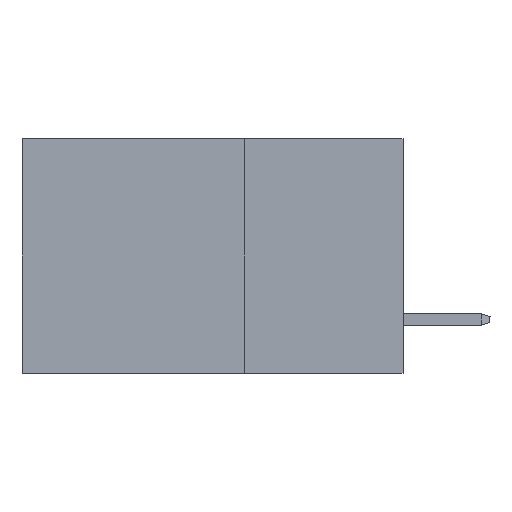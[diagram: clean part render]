
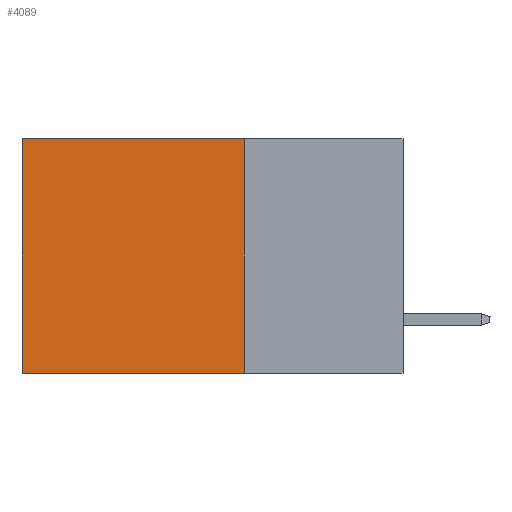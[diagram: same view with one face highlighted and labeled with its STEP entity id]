
A CAD part, left-side view. The second image highlights one B-rep face of the part: STEP entity #4089.
In plain terms, the highlighted planar face has unit normal (-1, 0, 0).
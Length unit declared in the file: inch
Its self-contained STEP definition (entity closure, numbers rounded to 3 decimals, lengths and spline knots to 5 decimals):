
#2768 = AXIS2_PLACEMENT_3D ( 'NONE', #8607, #30535, #14012 ) ;
#3609 = CARTESIAN_POINT ( 'NONE',  ( 0.2875, 0.6, 0. ) ) ;
#3750 = ORIENTED_EDGE ( 'NONE', *, *, #21855, .T. ) ;
#4089 = ADVANCED_FACE ( 'NONE', ( #13552 ), #20753, .F. ) ;
#5744 = CARTESIAN_POINT ( 'NONE',  ( 0.2875, 0.6, 0. ) ) ;
#6732 = CARTESIAN_POINT ( 'NONE',  ( 0.2875, 0.25, 0. ) ) ;
#8607 = CARTESIAN_POINT ( 'NONE',  ( 0.2875, 0.25, 0. ) ) ;
#8876 = EDGE_LOOP ( 'NONE', ( #3750, #11060, #24140, #12062 ) ) ;
#9125 = DIRECTION ( 'NONE',  ( 0., 0., -1. ) ) ;
#9235 = VERTEX_POINT ( 'NONE', #11275 ) ;
#9821 = DIRECTION ( 'NONE',  ( 0., 1., 0. ) ) ;
#10439 = EDGE_CURVE ( 'NONE', #28716, #9235, #26249, .T. ) ;
#11060 = ORIENTED_EDGE ( 'NONE', *, *, #17502, .F. ) ;
#11275 = CARTESIAN_POINT ( 'NONE',  ( 0.2875, 0.25, -0.37 ) ) ;
#11988 = CARTESIAN_POINT ( 'NONE',  ( 0.2875, 0.25, 0. ) ) ;
#12062 = ORIENTED_EDGE ( 'NONE', *, *, #19594, .T. ) ;
#13019 = VERTEX_POINT ( 'NONE', #29179 ) ;
#13552 = FACE_OUTER_BOUND ( 'NONE', #8876, .T. ) ;
#14012 = DIRECTION ( 'NONE',  ( 0., 0., -1. ) ) ;
#16333 = VECTOR ( 'NONE', #26515, 39.37008 ) ;
#17058 = LINE ( 'NONE', #19467, #16333 ) ;
#17502 = EDGE_CURVE ( 'NONE', #9235, #13019, #17058, .T. ) ;
#17762 = DIRECTION ( 'NONE',  ( 0., 0., -1. ) ) ;
#17910 = VECTOR ( 'NONE', #9821, 39.37008 ) ;
#19467 = CARTESIAN_POINT ( 'NONE',  ( 0.2875, 0.25, -0.37 ) ) ;
#19594 = EDGE_CURVE ( 'NONE', #28716, #25861, #26473, .T. ) ;
#20753 = PLANE ( 'NONE',  #2768 ) ;
#21829 = CARTESIAN_POINT ( 'NONE',  ( 0.2875, 0.25, 0. ) ) ;
#21855 = EDGE_CURVE ( 'NONE', #25861, #13019, #29934, .T. ) ;
#23632 = VECTOR ( 'NONE', #17762, 39.37008 ) ;
#24140 = ORIENTED_EDGE ( 'NONE', *, *, #10439, .F. ) ;
#25861 = VERTEX_POINT ( 'NONE', #3609 ) ;
#26249 = LINE ( 'NONE', #11988, #29777 ) ;
#26473 = LINE ( 'NONE', #21829, #17910 ) ;
#26515 = DIRECTION ( 'NONE',  ( 0., 1., 0. ) ) ;
#28716 = VERTEX_POINT ( 'NONE', #6732 ) ;
#29179 = CARTESIAN_POINT ( 'NONE',  ( 0.2875, 0.6, -0.37 ) ) ;
#29777 = VECTOR ( 'NONE', #9125, 39.37008 ) ;
#29934 = LINE ( 'NONE', #5744, #23632 ) ;
#30535 = DIRECTION ( 'NONE',  ( 1., 0., 0. ) ) ;
